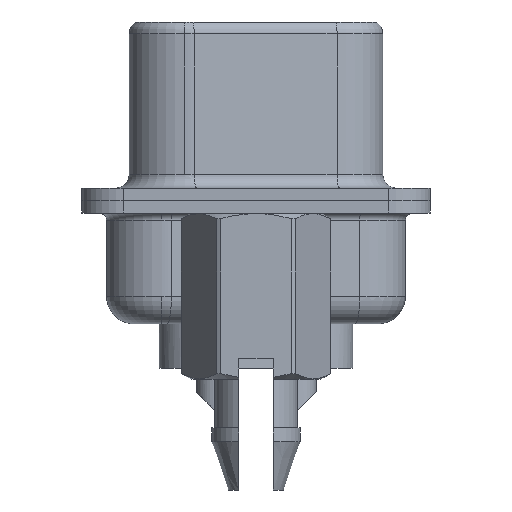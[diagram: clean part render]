
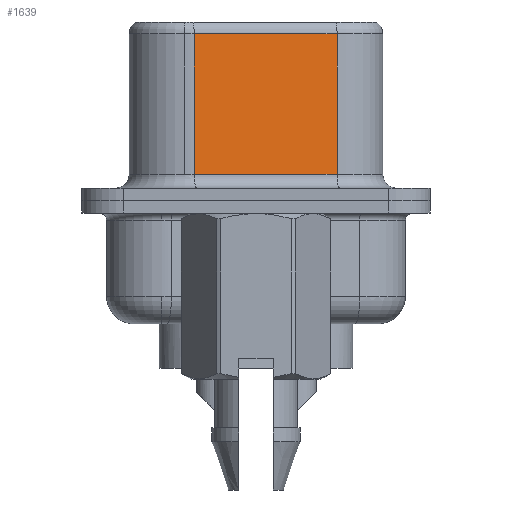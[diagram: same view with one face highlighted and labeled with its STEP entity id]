
A CAD part, left-side view. The second image highlights one B-rep face of the part: STEP entity #1639.
In plain terms, the highlighted planar face has unit normal (-0.985, -0.174, 0).
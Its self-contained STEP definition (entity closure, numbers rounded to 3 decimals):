
#455 = ORIENTED_EDGE ( 'NONE', *, *, #9094, .T. ) ;
#482 = VERTEX_POINT ( 'NONE', #9941 ) ;
#1000 = DIRECTION ( 'NONE',  ( 0., 0., -1. ) ) ;
#1639 = ADVANCED_FACE ( 'NONE', ( #13052 ), #15761, .F. ) ;
#1782 = DIRECTION ( 'NONE',  ( 0., 0., -1. ) ) ;
#1866 = VECTOR ( 'NONE', #6393, 1000. ) ;
#2567 = CARTESIAN_POINT ( 'NONE',  ( 3.665, 2.233, 6.52 ) ) ;
#3046 = CARTESIAN_POINT ( 'NONE',  ( 4.575, -2.927, 6.02 ) ) ;
#3428 = VECTOR ( 'NONE', #4605, 1000. ) ;
#4440 = LINE ( 'NONE', #3046, #3428 ) ;
#4605 = DIRECTION ( 'NONE',  ( -0.174, 0.985, 0. ) ) ;
#5130 = EDGE_CURVE ( 'NONE', #11588, #17135, #4440, .T. ) ;
#5436 = CARTESIAN_POINT ( 'NONE',  ( 3.665, 2.233, 0.95 ) ) ;
#6146 = CARTESIAN_POINT ( 'NONE',  ( 3.665, 2.233, 6.02 ) ) ;
#6393 = DIRECTION ( 'NONE',  ( 0.174, -0.985, 0. ) ) ;
#8503 = ORIENTED_EDGE ( 'NONE', *, *, #17200, .T. ) ;
#8520 = VECTOR ( 'NONE', #1000, 1000. ) ;
#9094 = EDGE_CURVE ( 'NONE', #17316, #482, #15266, .T. ) ;
#9480 = EDGE_LOOP ( 'NONE', ( #16924, #16959, #8503, #455 ) ) ;
#9513 = LINE ( 'NONE', #13539, #13947 ) ;
#9941 = CARTESIAN_POINT ( 'NONE',  ( 4.575, -2.927, 0.95 ) ) ;
#10497 = CARTESIAN_POINT ( 'NONE',  ( 4.575, -2.927, 6.52 ) ) ;
#11201 = AXIS2_PLACEMENT_3D ( 'NONE', #10497, #14880, #11908 ) ;
#11588 = VERTEX_POINT ( 'NONE', #13754 ) ;
#11755 = CARTESIAN_POINT ( 'NONE',  ( 4.575, -2.927, 0.95 ) ) ;
#11908 = DIRECTION ( 'NONE',  ( -0.174, 0.985, 0. ) ) ;
#12348 = EDGE_CURVE ( 'NONE', #11588, #482, #9513, .T. ) ;
#13052 = FACE_OUTER_BOUND ( 'NONE', #9480, .T. ) ;
#13539 = CARTESIAN_POINT ( 'NONE',  ( 4.575, -2.927, 6.52 ) ) ;
#13754 = CARTESIAN_POINT ( 'NONE',  ( 4.575, -2.927, 6.02 ) ) ;
#13947 = VECTOR ( 'NONE', #1782, 1000. ) ;
#14880 = DIRECTION ( 'NONE',  ( 0.985, 0.174, 0. ) ) ;
#15266 = LINE ( 'NONE', #11755, #1866 ) ;
#15761 = PLANE ( 'NONE',  #11201 ) ;
#16924 = ORIENTED_EDGE ( 'NONE', *, *, #12348, .F. ) ;
#16959 = ORIENTED_EDGE ( 'NONE', *, *, #5130, .T. ) ;
#17119 = LINE ( 'NONE', #2567, #8520 ) ;
#17135 = VERTEX_POINT ( 'NONE', #6146 ) ;
#17200 = EDGE_CURVE ( 'NONE', #17135, #17316, #17119, .T. ) ;
#17316 = VERTEX_POINT ( 'NONE', #5436 ) ;
